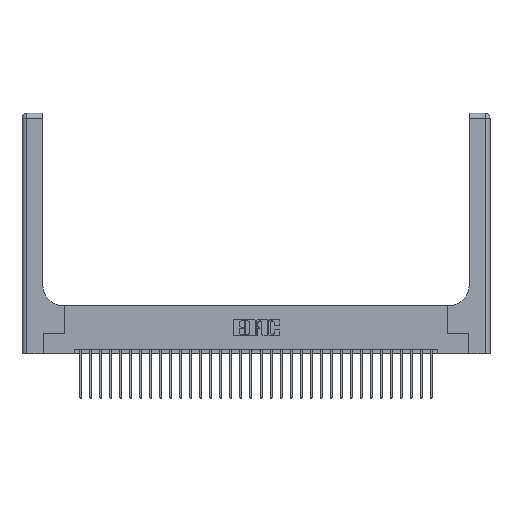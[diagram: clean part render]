
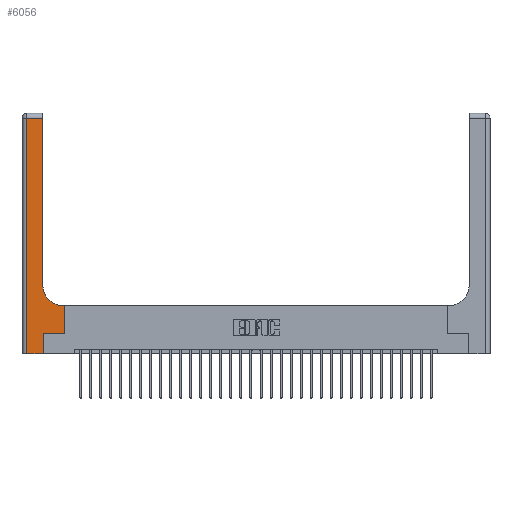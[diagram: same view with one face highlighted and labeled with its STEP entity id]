
A CAD part, top view. The second image highlights one B-rep face of the part: STEP entity #6056.
In plain terms, the highlighted planar face has unit normal (0, 0, 1).
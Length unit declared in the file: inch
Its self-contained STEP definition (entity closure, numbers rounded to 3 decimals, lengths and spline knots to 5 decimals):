
#106 = EDGE_CURVE ( 'NONE', #19083, #19833, #1053, .T. ) ;
#157 = CARTESIAN_POINT ( 'NONE',  ( 0.265, 0., 0.37 ) ) ;
#191 = DIRECTION ( 'NONE',  ( 0., 0., -1. ) ) ;
#1053 = LINE ( 'NONE', #13817, #24541 ) ;
#1226 = VECTOR ( 'NONE', #28505, 39.37008 ) ;
#1270 = VECTOR ( 'NONE', #5396, 39.37008 ) ;
#1284 = CARTESIAN_POINT ( 'NONE',  ( 0., 3., 0.37 ) ) ;
#1683 = AXIS2_PLACEMENT_3D ( 'NONE', #1284, #3585, #19806 ) ;
#1763 = CARTESIAN_POINT ( 'NONE',  ( 0.06, 2.94, 0.37 ) ) ;
#2001 = AXIS2_PLACEMENT_3D ( 'NONE', #9372, #191, #23097 ) ;
#3110 = CARTESIAN_POINT ( 'NONE',  ( 0.528, 0.25, 0.37 ) ) ;
#3585 = DIRECTION ( 'NONE',  ( 0., 0., -1. ) ) ;
#4928 = ORIENTED_EDGE ( 'NONE', *, *, #20371, .T. ) ;
#5387 = VERTEX_POINT ( 'NONE', #27541 ) ;
#5396 = DIRECTION ( 'NONE',  ( 0., 1., 0. ) ) ;
#5589 = ORIENTED_EDGE ( 'NONE', *, *, #11120, .T. ) ;
#6056 = ADVANCED_FACE ( 'NONE', ( #20117 ), #8049, .F. ) ;
#6954 = CARTESIAN_POINT ( 'NONE',  ( 0., 2.94, 0.37 ) ) ;
#6965 = CIRCLE ( 'NONE', #2001, 0.25 ) ;
#8049 = PLANE ( 'NONE',  #1683 ) ;
#8613 = EDGE_CURVE ( 'NONE', #12348, #19083, #9326, .T. ) ;
#8975 = VECTOR ( 'NONE', #22675, 39.37008 ) ;
#9326 = LINE ( 'NONE', #157, #8975 ) ;
#9372 = CARTESIAN_POINT ( 'NONE',  ( 0.51, 0.85, 0.37 ) ) ;
#9469 = CARTESIAN_POINT ( 'NONE',  ( 0.51, 0.6, 0.37 ) ) ;
#10415 = CARTESIAN_POINT ( 'NONE',  ( 0.06, 3., 0.37 ) ) ;
#10745 = ORIENTED_EDGE ( 'NONE', *, *, #17207, .T. ) ;
#10955 = VECTOR ( 'NONE', #11440, 39.37008 ) ;
#11120 = EDGE_CURVE ( 'NONE', #12529, #22275, #25161, .T. ) ;
#11222 = LINE ( 'NONE', #28421, #1226 ) ;
#11335 = CARTESIAN_POINT ( 'NONE',  ( 0.26, 3., 0.37 ) ) ;
#11440 = DIRECTION ( 'NONE',  ( -1., 0., 0. ) ) ;
#11520 = EDGE_CURVE ( 'NONE', #5387, #18462, #27554, .T. ) ;
#12160 = CARTESIAN_POINT ( 'NONE',  ( 0.265, 0., 0.37 ) ) ;
#12348 = VERTEX_POINT ( 'NONE', #12160 ) ;
#12529 = VERTEX_POINT ( 'NONE', #1763 ) ;
#12690 = DIRECTION ( 'NONE',  ( 0., -1., 0. ) ) ;
#13367 = VERTEX_POINT ( 'NONE', #9469 ) ;
#13396 = VECTOR ( 'NONE', #12690, 39.37008 ) ;
#13543 = EDGE_LOOP ( 'NONE', ( #20249, #4928, #5589, #26930, #17713, #15891, #24030, #15944, #10745 ) ) ;
#13817 = CARTESIAN_POINT ( 'NONE',  ( 0.265, 0.25, 0.37 ) ) ;
#14379 = VECTOR ( 'NONE', #20738, 39.37008 ) ;
#15891 = ORIENTED_EDGE ( 'NONE', *, *, #106, .T. ) ;
#15944 = ORIENTED_EDGE ( 'NONE', *, *, #22109, .T. ) ;
#16501 = VECTOR ( 'NONE', #20849, 39.37008 ) ;
#16824 = CARTESIAN_POINT ( 'NONE',  ( 0.528, 0.6, 0.37 ) ) ;
#17207 = EDGE_CURVE ( 'NONE', #13367, #5387, #6965, .T. ) ;
#17713 = ORIENTED_EDGE ( 'NONE', *, *, #8613, .T. ) ;
#18006 = LINE ( 'NONE', #3110, #1270 ) ;
#18462 = VERTEX_POINT ( 'NONE', #22549 ) ;
#18467 = CARTESIAN_POINT ( 'NONE',  ( 0.26, 0.6, 0.37 ) ) ;
#18651 = CARTESIAN_POINT ( 'NONE',  ( 0.06, 0., 0.37 ) ) ;
#19083 = VERTEX_POINT ( 'NONE', #27218 ) ;
#19435 = VERTEX_POINT ( 'NONE', #16824 ) ;
#19806 = DIRECTION ( 'NONE',  ( -1., 0., 0. ) ) ;
#19833 = VERTEX_POINT ( 'NONE', #22479 ) ;
#20117 = FACE_OUTER_BOUND ( 'NONE', #13543, .T. ) ;
#20249 = ORIENTED_EDGE ( 'NONE', *, *, #11520, .T. ) ;
#20371 = EDGE_CURVE ( 'NONE', #18462, #12529, #21260, .T. ) ;
#20738 = DIRECTION ( 'NONE',  ( -1., 0., 0. ) ) ;
#20849 = DIRECTION ( 'NONE',  ( 0., 1., 0. ) ) ;
#20994 = EDGE_CURVE ( 'NONE', #19833, #19435, #18006, .T. ) ;
#21260 = LINE ( 'NONE', #6954, #10955 ) ;
#22109 = EDGE_CURVE ( 'NONE', #19435, #13367, #26500, .T. ) ;
#22275 = VERTEX_POINT ( 'NONE', #18651 ) ;
#22479 = CARTESIAN_POINT ( 'NONE',  ( 0.528, 0.25, 0.37 ) ) ;
#22549 = CARTESIAN_POINT ( 'NONE',  ( 0.26, 2.94, 0.37 ) ) ;
#22675 = DIRECTION ( 'NONE',  ( 0., 1., 0. ) ) ;
#23097 = DIRECTION ( 'NONE',  ( 1., 0., 0. ) ) ;
#24030 = ORIENTED_EDGE ( 'NONE', *, *, #20994, .T. ) ;
#24541 = VECTOR ( 'NONE', #27495, 39.37008 ) ;
#25161 = LINE ( 'NONE', #10415, #13396 ) ;
#26500 = LINE ( 'NONE', #18467, #14379 ) ;
#26930 = ORIENTED_EDGE ( 'NONE', *, *, #28431, .T. ) ;
#27218 = CARTESIAN_POINT ( 'NONE',  ( 0.265, 0.25, 0.37 ) ) ;
#27495 = DIRECTION ( 'NONE',  ( 1., 0., 0. ) ) ;
#27541 = CARTESIAN_POINT ( 'NONE',  ( 0.26, 0.85, 0.37 ) ) ;
#27554 = LINE ( 'NONE', #11335, #16501 ) ;
#28421 = CARTESIAN_POINT ( 'NONE',  ( 0., 0., 0.37 ) ) ;
#28431 = EDGE_CURVE ( 'NONE', #22275, #12348, #11222, .T. ) ;
#28505 = DIRECTION ( 'NONE',  ( 1., 0., 0. ) ) ;
